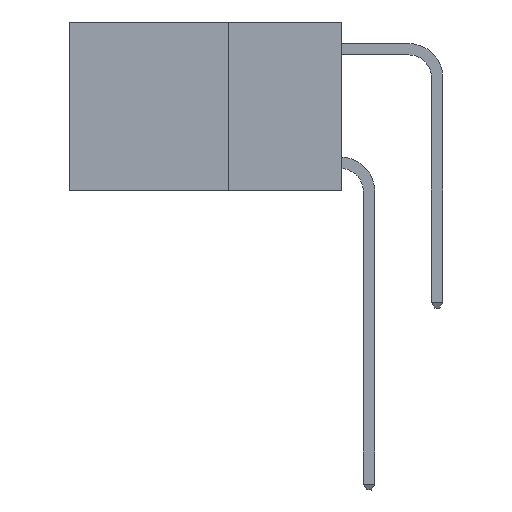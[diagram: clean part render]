
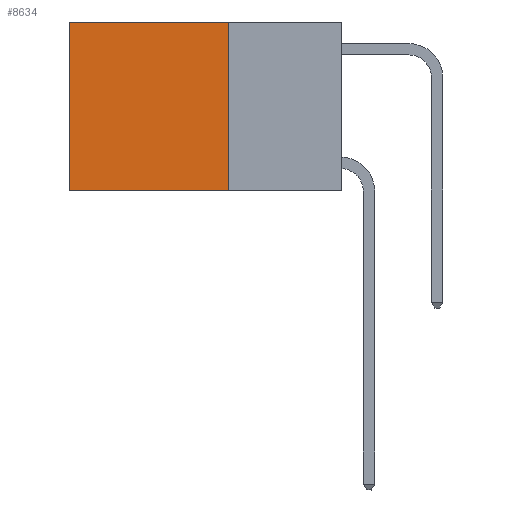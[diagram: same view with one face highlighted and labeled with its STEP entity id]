
A CAD part, left-side view. The second image highlights one B-rep face of the part: STEP entity #8634.
In plain terms, the highlighted planar face has unit normal (-1, 0, 0).
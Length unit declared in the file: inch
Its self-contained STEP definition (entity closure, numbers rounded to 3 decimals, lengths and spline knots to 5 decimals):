
#2 = VECTOR ( 'NONE', #16273, 39.37008 ) ;
#341 = ORIENTED_EDGE ( 'NONE', *, *, #13822, .T. ) ;
#573 = CARTESIAN_POINT ( 'NONE',  ( 0.2625, 0.6, 0. ) ) ;
#685 = LINE ( 'NONE', #8877, #4002 ) ;
#1159 = FACE_OUTER_BOUND ( 'NONE', #15822, .T. ) ;
#1497 = CARTESIAN_POINT ( 'NONE',  ( 0.2625, 0.25, 0. ) ) ;
#1676 = VERTEX_POINT ( 'NONE', #573 ) ;
#1819 = CARTESIAN_POINT ( 'NONE',  ( 0.2625, 0.6, -0.37 ) ) ;
#1946 = CARTESIAN_POINT ( 'NONE',  ( 0.2625, 0.25, -0.37 ) ) ;
#2114 = VECTOR ( 'NONE', #2408, 39.37008 ) ;
#2408 = DIRECTION ( 'NONE',  ( 0., 0., -1. ) ) ;
#2922 = DIRECTION ( 'NONE',  ( 0., 0., -1. ) ) ;
#3734 = VERTEX_POINT ( 'NONE', #1946 ) ;
#4002 = VECTOR ( 'NONE', #10263, 39.37008 ) ;
#4497 = VERTEX_POINT ( 'NONE', #1819 ) ;
#4684 = CARTESIAN_POINT ( 'NONE',  ( 0.2625, 0.25, -0.37 ) ) ;
#5234 = CARTESIAN_POINT ( 'NONE',  ( 0.2625, 0.6, 0. ) ) ;
#6107 = DIRECTION ( 'NONE',  ( 0., 1., 0. ) ) ;
#6409 = EDGE_CURVE ( 'NONE', #17547, #1676, #685, .T. ) ;
#6772 = CARTESIAN_POINT ( 'NONE',  ( 0.2625, 0.25, 0. ) ) ;
#7872 = ORIENTED_EDGE ( 'NONE', *, *, #10052, .F. ) ;
#8574 = PLANE ( 'NONE',  #17606 ) ;
#8634 = ADVANCED_FACE ( 'NONE', ( #1159 ), #8574, .F. ) ;
#8877 = CARTESIAN_POINT ( 'NONE',  ( 0.2625, 0.25, 0. ) ) ;
#9613 = LINE ( 'NONE', #5234, #2114 ) ;
#9725 = LINE ( 'NONE', #4684, #12479 ) ;
#9829 = ORIENTED_EDGE ( 'NONE', *, *, #6409, .T. ) ;
#10052 = EDGE_CURVE ( 'NONE', #3734, #4497, #9725, .T. ) ;
#10263 = DIRECTION ( 'NONE',  ( 0., 1., 0. ) ) ;
#11307 = DIRECTION ( 'NONE',  ( 1., 0., 0. ) ) ;
#12479 = VECTOR ( 'NONE', #6107, 39.37008 ) ;
#13822 = EDGE_CURVE ( 'NONE', #1676, #4497, #9613, .T. ) ;
#14203 = CARTESIAN_POINT ( 'NONE',  ( 0.2625, 0.25, 0. ) ) ;
#14340 = LINE ( 'NONE', #6772, #2 ) ;
#14948 = ORIENTED_EDGE ( 'NONE', *, *, #16619, .F. ) ;
#15822 = EDGE_LOOP ( 'NONE', ( #341, #7872, #14948, #9829 ) ) ;
#16273 = DIRECTION ( 'NONE',  ( 0., 0., -1. ) ) ;
#16619 = EDGE_CURVE ( 'NONE', #17547, #3734, #14340, .T. ) ;
#17547 = VERTEX_POINT ( 'NONE', #14203 ) ;
#17606 = AXIS2_PLACEMENT_3D ( 'NONE', #1497, #11307, #2922 ) ;
